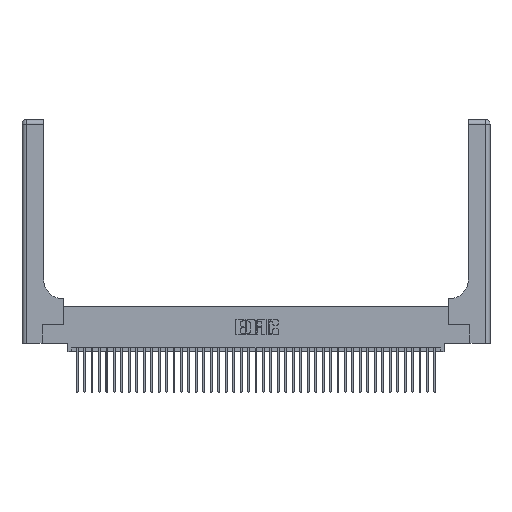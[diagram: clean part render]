
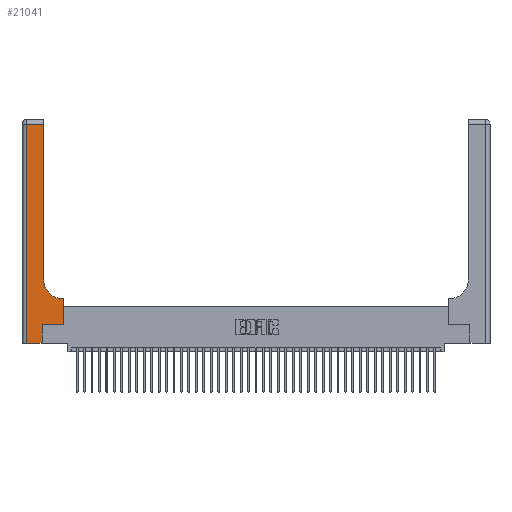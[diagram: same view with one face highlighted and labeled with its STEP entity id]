
A CAD part, top view. The second image highlights one B-rep face of the part: STEP entity #21041.
In plain terms, the highlighted planar face has unit normal (0, 0, 1).
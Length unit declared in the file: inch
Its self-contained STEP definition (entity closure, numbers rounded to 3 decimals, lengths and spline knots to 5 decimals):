
#283 = VECTOR ( 'NONE', #17033, 39.37008 ) ;
#350 = EDGE_CURVE ( 'NONE', #38507, #37595, #12857, .T. ) ;
#1009 = CARTESIAN_POINT ( 'NONE',  ( 0., 2.94, 0.37 ) ) ;
#1059 = DIRECTION ( 'NONE',  ( 0., 0., -1. ) ) ;
#1542 = ORIENTED_EDGE ( 'NONE', *, *, #16832, .T. ) ;
#1646 = EDGE_CURVE ( 'NONE', #38271, #7137, #16932, .T. ) ;
#2205 = DIRECTION ( 'NONE',  ( 0., 1., 0. ) ) ;
#2278 = VECTOR ( 'NONE', #15481, 39.37008 ) ;
#4350 = LINE ( 'NONE', #1009, #37437 ) ;
#4373 = LINE ( 'NONE', #12096, #2278 ) ;
#4468 = CARTESIAN_POINT ( 'NONE',  ( 0.269, 0.25, 0.37 ) ) ;
#4502 = DIRECTION ( 'NONE',  ( -1., 0., 0. ) ) ;
#4857 = EDGE_CURVE ( 'NONE', #7137, #29931, #4373, .T. ) ;
#5336 = ORIENTED_EDGE ( 'NONE', *, *, #42222, .T. ) ;
#5842 = ORIENTED_EDGE ( 'NONE', *, *, #42078, .T. ) ;
#5866 = CARTESIAN_POINT ( 'NONE',  ( 0.5585, 0.25, 0.37 ) ) ;
#6650 = EDGE_CURVE ( 'NONE', #8819, #38507, #33158, .T. ) ;
#6717 = ORIENTED_EDGE ( 'NONE', *, *, #1646, .T. ) ;
#6951 = PLANE ( 'NONE',  #15265 ) ;
#7137 = VERTEX_POINT ( 'NONE', #33316 ) ;
#7944 = VERTEX_POINT ( 'NONE', #4468 ) ;
#8819 = VERTEX_POINT ( 'NONE', #5866 ) ;
#9714 = ORIENTED_EDGE ( 'NONE', *, *, #26883, .T. ) ;
#12043 = ORIENTED_EDGE ( 'NONE', *, *, #6650, .T. ) ;
#12096 = CARTESIAN_POINT ( 'NONE',  ( 0., 0., 0.37 ) ) ;
#12105 = CARTESIAN_POINT ( 'NONE',  ( 0.269, 0., 0.37 ) ) ;
#12163 = CARTESIAN_POINT ( 'NONE',  ( 0.2915, 3., 0.37 ) ) ;
#12857 = LINE ( 'NONE', #23285, #32403 ) ;
#13670 = ORIENTED_EDGE ( 'NONE', *, *, #350, .T. ) ;
#13689 = CARTESIAN_POINT ( 'NONE',  ( 0.269, 0.25, 0.37 ) ) ;
#15265 = AXIS2_PLACEMENT_3D ( 'NONE', #17047, #40009, #20303 ) ;
#15481 = DIRECTION ( 'NONE',  ( 1., 0., 0. ) ) ;
#16578 = CARTESIAN_POINT ( 'NONE',  ( 0.5585, 0.25, 0.37 ) ) ;
#16832 = EDGE_CURVE ( 'NONE', #29931, #7944, #22649, .T. ) ;
#16895 = DIRECTION ( 'NONE',  ( -1., 0., 0. ) ) ;
#16930 = CARTESIAN_POINT ( 'NONE',  ( 0.269, 0., 0.37 ) ) ;
#16932 = LINE ( 'NONE', #25411, #41073 ) ;
#17033 = DIRECTION ( 'NONE',  ( 1., 0., 0. ) ) ;
#17047 = CARTESIAN_POINT ( 'NONE',  ( 0., 3., 0.37 ) ) ;
#17408 = CARTESIAN_POINT ( 'NONE',  ( 0.5585, 0.6, 0.37 ) ) ;
#20190 = DIRECTION ( 'NONE',  ( 0., 1., 0. ) ) ;
#20303 = DIRECTION ( 'NONE',  ( -1., 0., 0. ) ) ;
#20980 = CARTESIAN_POINT ( 'NONE',  ( 0.5415, 0.85, 0.37 ) ) ;
#21041 = ADVANCED_FACE ( 'NONE', ( #24833 ), #6951, .F. ) ;
#22082 = LINE ( 'NONE', #12163, #38543 ) ;
#22183 = VERTEX_POINT ( 'NONE', #35384 ) ;
#22649 = LINE ( 'NONE', #16930, #39130 ) ;
#23285 = CARTESIAN_POINT ( 'NONE',  ( 0.2915, 0.6, 0.37 ) ) ;
#23978 = EDGE_LOOP ( 'NONE', ( #24638, #9714, #6717, #40862, #1542, #5842, #12043, #13670, #5336 ) ) ;
#24264 = DIRECTION ( 'NONE',  ( 1., 0., 0. ) ) ;
#24396 = VECTOR ( 'NONE', #39543, 39.37008 ) ;
#24638 = ORIENTED_EDGE ( 'NONE', *, *, #42446, .T. ) ;
#24833 = FACE_OUTER_BOUND ( 'NONE', #23978, .T. ) ;
#25411 = CARTESIAN_POINT ( 'NONE',  ( 0.06, 3., 0.37 ) ) ;
#26731 = LINE ( 'NONE', #13689, #283 ) ;
#26883 = EDGE_CURVE ( 'NONE', #27519, #38271, #4350, .T. ) ;
#27519 = VERTEX_POINT ( 'NONE', #33803 ) ;
#29931 = VERTEX_POINT ( 'NONE', #12105 ) ;
#31947 = CARTESIAN_POINT ( 'NONE',  ( 0.5415, 0.6, 0.37 ) ) ;
#32044 = DIRECTION ( 'NONE',  ( 0., -1., 0. ) ) ;
#32403 = VECTOR ( 'NONE', #16895, 39.37008 ) ;
#33158 = LINE ( 'NONE', #16578, #24396 ) ;
#33316 = CARTESIAN_POINT ( 'NONE',  ( 0.06, 0., 0.37 ) ) ;
#33803 = CARTESIAN_POINT ( 'NONE',  ( 0.2915, 2.94, 0.37 ) ) ;
#35384 = CARTESIAN_POINT ( 'NONE',  ( 0.2915, 0.85, 0.37 ) ) ;
#35735 = CARTESIAN_POINT ( 'NONE',  ( 0.06, 2.94, 0.37 ) ) ;
#37437 = VECTOR ( 'NONE', #4502, 39.37008 ) ;
#37595 = VERTEX_POINT ( 'NONE', #31947 ) ;
#38029 = CIRCLE ( 'NONE', #40020, 0.25 ) ;
#38271 = VERTEX_POINT ( 'NONE', #35735 ) ;
#38507 = VERTEX_POINT ( 'NONE', #17408 ) ;
#38543 = VECTOR ( 'NONE', #2205, 39.37008 ) ;
#39130 = VECTOR ( 'NONE', #20190, 39.37008 ) ;
#39543 = DIRECTION ( 'NONE',  ( 0., 1., 0. ) ) ;
#40009 = DIRECTION ( 'NONE',  ( 0., 0., -1. ) ) ;
#40020 = AXIS2_PLACEMENT_3D ( 'NONE', #20980, #1059, #24264 ) ;
#40862 = ORIENTED_EDGE ( 'NONE', *, *, #4857, .T. ) ;
#41073 = VECTOR ( 'NONE', #32044, 39.37008 ) ;
#42078 = EDGE_CURVE ( 'NONE', #7944, #8819, #26731, .T. ) ;
#42222 = EDGE_CURVE ( 'NONE', #37595, #22183, #38029, .T. ) ;
#42446 = EDGE_CURVE ( 'NONE', #22183, #27519, #22082, .T. ) ;
